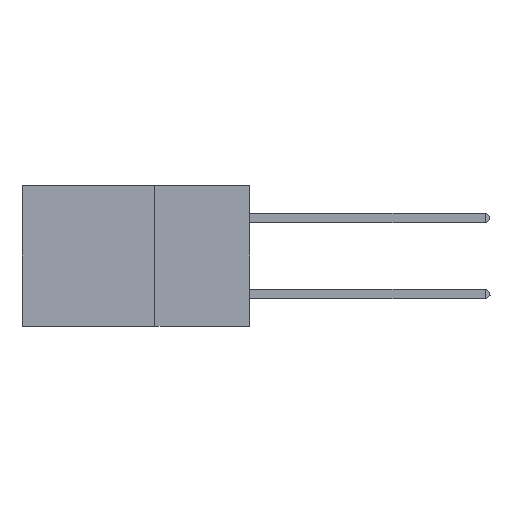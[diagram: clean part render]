
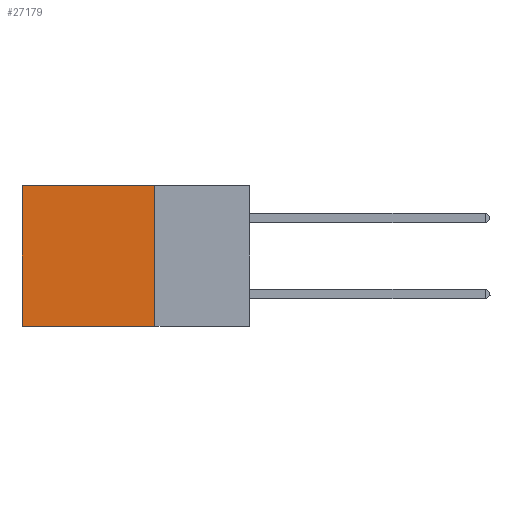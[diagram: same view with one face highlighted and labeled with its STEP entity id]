
A CAD part, left-side view. The second image highlights one B-rep face of the part: STEP entity #27179.
In plain terms, the highlighted planar face has unit normal (-1, 0, 0).
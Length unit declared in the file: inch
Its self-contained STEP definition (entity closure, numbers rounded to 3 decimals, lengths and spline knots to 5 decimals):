
#243 = EDGE_CURVE ( 'NONE', #9305, #24728, #11742, .T. ) ;
#1232 = LINE ( 'NONE', #21541, #30850 ) ;
#1654 = VERTEX_POINT ( 'NONE', #11667 ) ;
#1682 = CARTESIAN_POINT ( 'NONE',  ( 0.2875, 0.25, 0. ) ) ;
#2512 = DIRECTION ( 'NONE',  ( 0., 0., -1. ) ) ;
#2627 = DIRECTION ( 'NONE',  ( 0., 0., -1. ) ) ;
#4240 = FACE_OUTER_BOUND ( 'NONE', #29241, .T. ) ;
#5734 = EDGE_CURVE ( 'NONE', #14259, #24728, #1232, .T. ) ;
#6484 = DIRECTION ( 'NONE',  ( 0., 1., 0. ) ) ;
#7627 = VECTOR ( 'NONE', #16623, 39.37008 ) ;
#8032 = LINE ( 'NONE', #1682, #16606 ) ;
#8526 = CARTESIAN_POINT ( 'NONE',  ( 0.2875, 0.6, -0.37 ) ) ;
#8671 = AXIS2_PLACEMENT_3D ( 'NONE', #11794, #26535, #2512 ) ;
#9305 = VERTEX_POINT ( 'NONE', #22633 ) ;
#9608 = CARTESIAN_POINT ( 'NONE',  ( 0.2875, 0.6, 0. ) ) ;
#11317 = EDGE_CURVE ( 'NONE', #1654, #14259, #8032, .T. ) ;
#11667 = CARTESIAN_POINT ( 'NONE',  ( 0.2875, 0.25, 0. ) ) ;
#11742 = LINE ( 'NONE', #19121, #7627 ) ;
#11794 = CARTESIAN_POINT ( 'NONE',  ( 0.2875, 0.25, 0. ) ) ;
#13639 = DIRECTION ( 'NONE',  ( 0., 0., -1. ) ) ;
#14259 = VERTEX_POINT ( 'NONE', #9608 ) ;
#14607 = LINE ( 'NONE', #16871, #21662 ) ;
#16289 = EDGE_CURVE ( 'NONE', #1654, #9305, #14607, .T. ) ;
#16606 = VECTOR ( 'NONE', #6484, 39.37008 ) ;
#16623 = DIRECTION ( 'NONE',  ( 0., 1., 0. ) ) ;
#16871 = CARTESIAN_POINT ( 'NONE',  ( 0.2875, 0.25, 0. ) ) ;
#16958 = PLANE ( 'NONE',  #8671 ) ;
#17923 = ORIENTED_EDGE ( 'NONE', *, *, #243, .F. ) ;
#19121 = CARTESIAN_POINT ( 'NONE',  ( 0.2875, 0.25, -0.37 ) ) ;
#21541 = CARTESIAN_POINT ( 'NONE',  ( 0.2875, 0.6, 0. ) ) ;
#21662 = VECTOR ( 'NONE', #2627, 39.37008 ) ;
#22633 = CARTESIAN_POINT ( 'NONE',  ( 0.2875, 0.25, -0.37 ) ) ;
#24728 = VERTEX_POINT ( 'NONE', #8526 ) ;
#25032 = ORIENTED_EDGE ( 'NONE', *, *, #5734, .T. ) ;
#25043 = ORIENTED_EDGE ( 'NONE', *, *, #11317, .T. ) ;
#26535 = DIRECTION ( 'NONE',  ( 1., 0., 0. ) ) ;
#27179 = ADVANCED_FACE ( 'NONE', ( #4240 ), #16958, .F. ) ;
#29241 = EDGE_LOOP ( 'NONE', ( #25032, #17923, #30131, #25043 ) ) ;
#30131 = ORIENTED_EDGE ( 'NONE', *, *, #16289, .F. ) ;
#30850 = VECTOR ( 'NONE', #13639, 39.37008 ) ;
